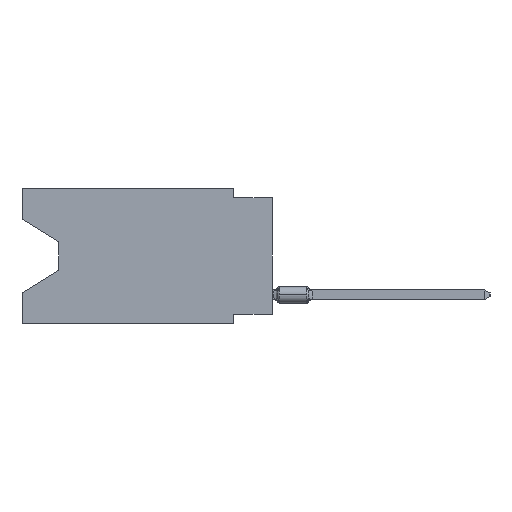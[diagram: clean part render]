
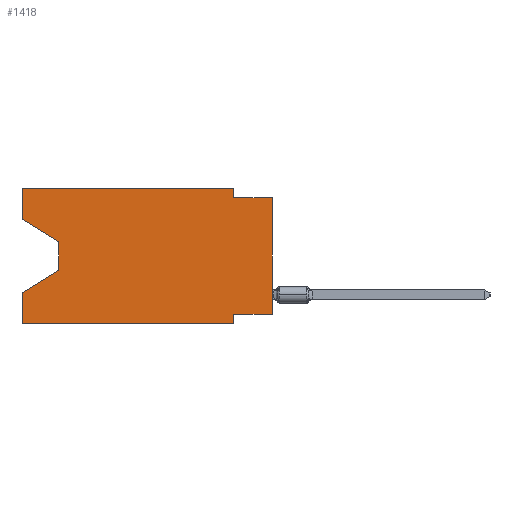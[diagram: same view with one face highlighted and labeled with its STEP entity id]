
A CAD part, left-side view. The second image highlights one B-rep face of the part: STEP entity #1418.
In plain terms, the highlighted planar face has unit normal (-1, 0, 0).
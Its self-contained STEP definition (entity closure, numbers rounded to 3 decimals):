
#204 = VECTOR ( 'NONE', #2364, 1000. ) ;
#411 = CARTESIAN_POINT ( 'NONE',  ( 0., 16.383, 0. ) ) ;
#604 = CARTESIAN_POINT ( 'NONE',  ( 0., 2.54, -8.255 ) ) ;
#708 = VERTEX_POINT ( 'NONE', #12155 ) ;
#1255 = DIRECTION ( 'NONE',  ( 0., 1., 0. ) ) ;
#1371 = VECTOR ( 'NONE', #14839, 1000. ) ;
#1418 = ADVANCED_FACE ( 'NONE', ( #17954 ), #20236, .F. ) ;
#1726 = VECTOR ( 'NONE', #31463, 1000. ) ;
#2364 = DIRECTION ( 'NONE',  ( 0., 0., 1. ) ) ;
#2519 = EDGE_LOOP ( 'NONE', ( #7726, #6649, #3995, #3533, #20361, #23241, #14214, #6539, #27506, #9193, #19299, #24744 ) ) ;
#2726 = CARTESIAN_POINT ( 'NONE',  ( 0., 13.97, -5.385 ) ) ;
#3533 = ORIENTED_EDGE ( 'NONE', *, *, #25893, .F. ) ;
#3682 = LINE ( 'NONE', #28313, #17099 ) ;
#3973 = DIRECTION ( 'NONE',  ( 0., 0., -1. ) ) ;
#3995 = ORIENTED_EDGE ( 'NONE', *, *, #8487, .T. ) ;
#4628 = LINE ( 'NONE', #22305, #1371 ) ;
#4953 = LINE ( 'NONE', #12421, #204 ) ;
#5787 = CARTESIAN_POINT ( 'NONE',  ( 0., 0., -0.635 ) ) ;
#6088 = EDGE_CURVE ( 'NONE', #14786, #9864, #9626, .T. ) ;
#6361 = EDGE_CURVE ( 'NONE', #29316, #14786, #26291, .T. ) ;
#6539 = ORIENTED_EDGE ( 'NONE', *, *, #17550, .T. ) ;
#6649 = ORIENTED_EDGE ( 'NONE', *, *, #10867, .T. ) ;
#6834 = VECTOR ( 'NONE', #10191, 1000. ) ;
#7026 = CARTESIAN_POINT ( 'NONE',  ( 0., 0., -8.255 ) ) ;
#7355 = DIRECTION ( 'NONE',  ( 0., -1., 0. ) ) ;
#7481 = VECTOR ( 'NONE', #10463, 1000. ) ;
#7726 = ORIENTED_EDGE ( 'NONE', *, *, #19939, .T. ) ;
#7995 = EDGE_CURVE ( 'NONE', #24877, #29316, #31973, .T. ) ;
#8349 = LINE ( 'NONE', #411, #7481 ) ;
#8487 = EDGE_CURVE ( 'NONE', #18043, #24445, #31062, .T. ) ;
#9193 = ORIENTED_EDGE ( 'NONE', *, *, #6361, .F. ) ;
#9247 = AXIS2_PLACEMENT_3D ( 'NONE', #22669, #31028, #3973 ) ;
#9550 = LINE ( 'NONE', #27195, #6834 ) ;
#9626 = LINE ( 'NONE', #19518, #27071 ) ;
#9755 = LINE ( 'NONE', #31781, #11763 ) ;
#9864 = VERTEX_POINT ( 'NONE', #5787 ) ;
#10129 = VECTOR ( 'NONE', #14046, 1000. ) ;
#10191 = DIRECTION ( 'NONE',  ( 0., 0., -1. ) ) ;
#10246 = EDGE_CURVE ( 'NONE', #708, #24877, #8349, .T. ) ;
#10463 = DIRECTION ( 'NONE',  ( 0., 0., 1. ) ) ;
#10867 = EDGE_CURVE ( 'NONE', #25825, #18043, #16779, .T. ) ;
#11302 = CARTESIAN_POINT ( 'NONE',  ( 0., 13.97, -3.505 ) ) ;
#11763 = VECTOR ( 'NONE', #14465, 1000. ) ;
#12155 = CARTESIAN_POINT ( 'NONE',  ( 0., 16.383, -2.038 ) ) ;
#12421 = CARTESIAN_POINT ( 'NONE',  ( 0., 16.383, 0. ) ) ;
#12693 = DIRECTION ( 'NONE',  ( 0., -1., 0. ) ) ;
#13091 = CARTESIAN_POINT ( 'NONE',  ( 0., 13.97, -5.385 ) ) ;
#13986 = CARTESIAN_POINT ( 'NONE',  ( 0., 2.54, 0. ) ) ;
#14046 = DIRECTION ( 'NONE',  ( 0., 0., -1. ) ) ;
#14214 = ORIENTED_EDGE ( 'NONE', *, *, #30233, .F. ) ;
#14465 = DIRECTION ( 'NONE',  ( 0., 0., 1. ) ) ;
#14786 = VERTEX_POINT ( 'NONE', #17986 ) ;
#14839 = DIRECTION ( 'NONE',  ( 0., -0.855, -0.519 ) ) ;
#15055 = VECTOR ( 'NONE', #16283, 1000. ) ;
#15680 = DIRECTION ( 'NONE',  ( 0., 0.855, -0.519 ) ) ;
#15894 = VERTEX_POINT ( 'NONE', #7026 ) ;
#16283 = DIRECTION ( 'NONE',  ( 0., -1., 0. ) ) ;
#16297 = CARTESIAN_POINT ( 'NONE',  ( 0., 2.54, 0. ) ) ;
#16402 = VERTEX_POINT ( 'NONE', #604 ) ;
#16626 = VERTEX_POINT ( 'NONE', #28626 ) ;
#16779 = LINE ( 'NONE', #21184, #10129 ) ;
#17099 = VECTOR ( 'NONE', #1255, 1000. ) ;
#17230 = CARTESIAN_POINT ( 'NONE',  ( 0., 16.383, 0. ) ) ;
#17466 = CARTESIAN_POINT ( 'NONE',  ( 0., 16.383, -6.852 ) ) ;
#17550 = EDGE_CURVE ( 'NONE', #15894, #9864, #9755, .T. ) ;
#17954 = FACE_OUTER_BOUND ( 'NONE', #2519, .T. ) ;
#17986 = CARTESIAN_POINT ( 'NONE',  ( 0., 2.54, -0.635 ) ) ;
#18043 = VERTEX_POINT ( 'NONE', #2726 ) ;
#19299 = ORIENTED_EDGE ( 'NONE', *, *, #7995, .F. ) ;
#19354 = CARTESIAN_POINT ( 'NONE',  ( 0., 16.383, -8.89 ) ) ;
#19518 = CARTESIAN_POINT ( 'NONE',  ( 0., 0., -0.635 ) ) ;
#19939 = EDGE_CURVE ( 'NONE', #708, #25825, #4628, .T. ) ;
#20236 = PLANE ( 'NONE',  #9247 ) ;
#20361 = ORIENTED_EDGE ( 'NONE', *, *, #26454, .T. ) ;
#20792 = CARTESIAN_POINT ( 'NONE',  ( 0., 16.383, 0. ) ) ;
#21184 = CARTESIAN_POINT ( 'NONE',  ( 0., 13.97, -3.505 ) ) ;
#21386 = VECTOR ( 'NONE', #12693, 1000. ) ;
#22305 = CARTESIAN_POINT ( 'NONE',  ( 0., 16.383, -2.038 ) ) ;
#22669 = CARTESIAN_POINT ( 'NONE',  ( 0., 16.383, 0. ) ) ;
#23241 = ORIENTED_EDGE ( 'NONE', *, *, #27359, .F. ) ;
#24445 = VERTEX_POINT ( 'NONE', #17466 ) ;
#24744 = ORIENTED_EDGE ( 'NONE', *, *, #10246, .F. ) ;
#24877 = VERTEX_POINT ( 'NONE', #20792 ) ;
#25825 = VERTEX_POINT ( 'NONE', #11302 ) ;
#25893 = EDGE_CURVE ( 'NONE', #16626, #24445, #4953, .T. ) ;
#26291 = LINE ( 'NONE', #13986, #1726 ) ;
#26454 = EDGE_CURVE ( 'NONE', #16626, #29328, #29072, .T. ) ;
#27071 = VECTOR ( 'NONE', #7355, 1000. ) ;
#27195 = CARTESIAN_POINT ( 'NONE',  ( 0., 2.54, -8.89 ) ) ;
#27359 = EDGE_CURVE ( 'NONE', #16402, #29328, #9550, .T. ) ;
#27506 = ORIENTED_EDGE ( 'NONE', *, *, #6088, .F. ) ;
#28313 = CARTESIAN_POINT ( 'NONE',  ( 0., 0., -8.255 ) ) ;
#28626 = CARTESIAN_POINT ( 'NONE',  ( 0., 16.383, -8.89 ) ) ;
#28927 = CARTESIAN_POINT ( 'NONE',  ( 0., 2.54, -8.89 ) ) ;
#29072 = LINE ( 'NONE', #19354, #15055 ) ;
#29316 = VERTEX_POINT ( 'NONE', #16297 ) ;
#29328 = VERTEX_POINT ( 'NONE', #28927 ) ;
#30179 = VECTOR ( 'NONE', #15680, 1000. ) ;
#30233 = EDGE_CURVE ( 'NONE', #15894, #16402, #3682, .T. ) ;
#31028 = DIRECTION ( 'NONE',  ( 1., 0., 0. ) ) ;
#31062 = LINE ( 'NONE', #13091, #30179 ) ;
#31463 = DIRECTION ( 'NONE',  ( 0., 0., -1. ) ) ;
#31781 = CARTESIAN_POINT ( 'NONE',  ( 0., 0., 0. ) ) ;
#31973 = LINE ( 'NONE', #17230, #21386 ) ;
